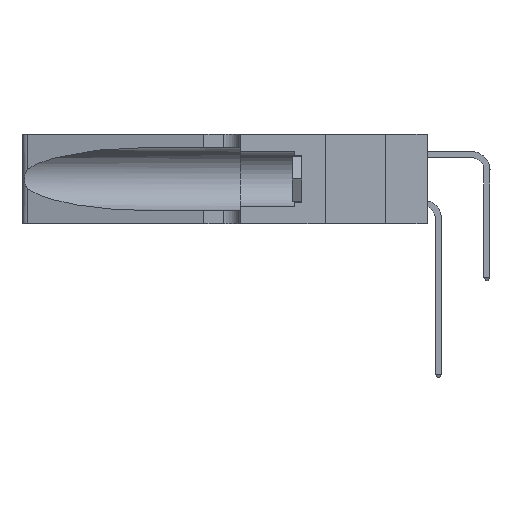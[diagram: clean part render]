
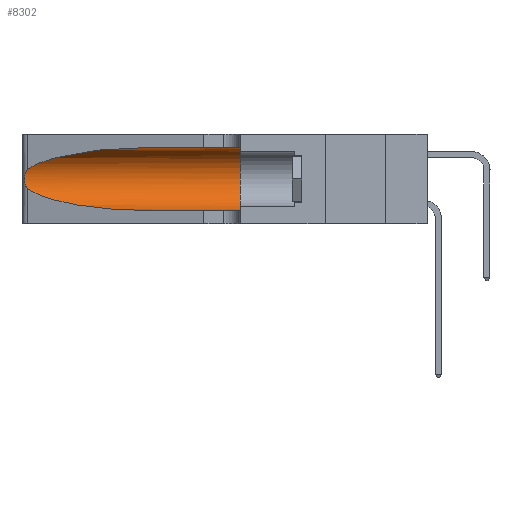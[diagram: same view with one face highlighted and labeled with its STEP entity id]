
A CAD part, left-side view. The second image highlights one B-rep face of the part: STEP entity #8302.
In plain terms, the highlighted cylindrical face has radius 3.308 mm (diameter 6.617 mm), a partial arc.
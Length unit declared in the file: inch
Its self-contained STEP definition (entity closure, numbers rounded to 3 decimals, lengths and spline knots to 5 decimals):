
#265 = EDGE_CURVE ( 'NONE', #23849, #14265, #804, .T. ) ;
#804 = B_SPLINE_CURVE_WITH_KNOTS ( 'NONE', 3,
 ( #3368, #3269, #7591, #3452, #15651, #3082, #5908, #24803, #11977, #8037, #22617, #1766, #9772, #3623 ),
 .UNSPECIFIED., .F., .F.,
 ( 4, 2, 2, 2, 2, 2, 4 ),
 ( 0., 0.00027, 0.00053, 0.00107, 0.0016, 0.00187, 0.00214 ),
 .UNSPECIFIED. ) ;
#1164 = CARTESIAN_POINT ( 'NONE',  ( 0.25487, 1.22718, 0.14631 ) ) ;
#1192 = DIRECTION ( 'NONE',  ( 0., -1., 0. ) ) ;
#1671 =( BOUNDED_CURVE ( )  B_SPLINE_CURVE ( 3, ( #26950, #3852, #14055, #14253 ),
 .UNSPECIFIED., .F., .T. ) 
 B_SPLINE_CURVE_WITH_KNOTS ( ( 4, 4 ),
 ( 1.5708, 2.84003 ),
 .UNSPECIFIED. ) 
 CURVE ( )  GEOMETRIC_REPRESENTATION_ITEM ( )  RATIONAL_B_SPLINE_CURVE ( ( 1., 0.87, 0.87, 1. ) ) 
 REPRESENTATION_ITEM ( '' )  );
#1766 = CARTESIAN_POINT ( 'NONE',  ( 0.25639, 1.23186, 0.15144 ) ) ;
#2797 = DIRECTION ( 'NONE',  ( 0., -1., 0. ) ) ;
#3082 = CARTESIAN_POINT ( 'NONE',  ( 0.26018, 1.23835, 0.19895 ) ) ;
#3269 = CARTESIAN_POINT ( 'NONE',  ( 0.25555, 1.22994, 0.2215 ) ) ;
#3368 = CARTESIAN_POINT ( 'NONE',  ( 0.25487, 1.22718, 0.22369 ) ) ;
#3452 = CARTESIAN_POINT ( 'NONE',  ( 0.25787, 1.23484, 0.2124 ) ) ;
#3623 = CARTESIAN_POINT ( 'NONE',  ( 0.25487, 1.22718, 0.14631 ) ) ;
#3852 = CARTESIAN_POINT ( 'NONE',  ( 0.18966, 0.96281, 0.31525 ) ) ;
#4766 = CARTESIAN_POINT ( 'NONE',  ( 0.1305, 0.72297, 0.31525 ) ) ;
#5136 = EDGE_CURVE ( 'NONE', #15925, #10423, #9144, .T. ) ;
#5548 = DIRECTION ( 'NONE',  ( 0., -1., 0. ) ) ;
#5908 = CARTESIAN_POINT ( 'NONE',  ( 0.26075, 1.23896, 0.19203 ) ) ;
#5994 = CYLINDRICAL_SURFACE ( 'NONE', #14311, 0.13025 ) ;
#6439 = CARTESIAN_POINT ( 'NONE',  ( 0.25487, 1.22718, 0.22369 ) ) ;
#6598 = EDGE_CURVE ( 'NONE', #14265, #10697, #26381, .T. ) ;
#7128 = CARTESIAN_POINT ( 'NONE',  ( 0.1305, 1.61858, 0.05475 ) ) ;
#7591 = CARTESIAN_POINT ( 'NONE',  ( 0.25639, 1.23184, 0.21858 ) ) ;
#8037 = CARTESIAN_POINT ( 'NONE',  ( 0.25856, 1.23593, 0.16098 ) ) ;
#8302 = ADVANCED_FACE ( 'NONE', ( #24354 ), #5994, .F. ) ;
#8969 = DIRECTION ( 'NONE',  ( 0., 1., 0. ) ) ;
#8988 = EDGE_CURVE ( 'NONE', #13413, #15925, #23983, .T. ) ;
#9144 = CIRCLE ( 'NONE', #11967, 0.13025 ) ;
#9772 = CARTESIAN_POINT ( 'NONE',  ( 0.25555, 1.22993, 0.14849 ) ) ;
#9868 = DIRECTION ( 'NONE',  ( 0., 0., -1. ) ) ;
#10423 = VERTEX_POINT ( 'NONE', #21136 ) ;
#10697 = VERTEX_POINT ( 'NONE', #17449 ) ;
#10906 = EDGE_CURVE ( 'NONE', #10697, #10423, #22584, .T. ) ;
#10915 = ORIENTED_EDGE ( 'NONE', *, *, #5136, .F. ) ;
#11065 = DIRECTION ( 'NONE',  ( 0., 0., 1. ) ) ;
#11659 = CARTESIAN_POINT ( 'NONE',  ( 0.18966, 0.96281, 0.05475 ) ) ;
#11967 = AXIS2_PLACEMENT_3D ( 'NONE', #23696, #8969, #11065 ) ;
#11977 = CARTESIAN_POINT ( 'NONE',  ( 0.26017, 1.23833, 0.17102 ) ) ;
#13413 = VERTEX_POINT ( 'NONE', #4766 ) ;
#13703 = EDGE_LOOP ( 'NONE', ( #15768, #22100, #19362, #14363, #10915, #14039 ) ) ;
#13873 = CARTESIAN_POINT ( 'NONE',  ( 0.1305, 1.61858, 0.31525 ) ) ;
#14039 = ORIENTED_EDGE ( 'NONE', *, *, #8988, .F. ) ;
#14055 = CARTESIAN_POINT ( 'NONE',  ( 0.2373, 1.15595, 0.28018 ) ) ;
#14253 = CARTESIAN_POINT ( 'NONE',  ( 0.25487, 1.22718, 0.22369 ) ) ;
#14265 = VERTEX_POINT ( 'NONE', #1164 ) ;
#14311 = AXIS2_PLACEMENT_3D ( 'NONE', #20161, #5548, #9868 ) ;
#14363 = ORIENTED_EDGE ( 'NONE', *, *, #10906, .T. ) ;
#15598 = CARTESIAN_POINT ( 'NONE',  ( 0.25487, 1.22718, 0.14631 ) ) ;
#15651 = CARTESIAN_POINT ( 'NONE',  ( 0.25854, 1.2359, 0.20912 ) ) ;
#15768 = ORIENTED_EDGE ( 'NONE', *, *, #23073, .T. ) ;
#15925 = VERTEX_POINT ( 'NONE', #24292 ) ;
#17449 = CARTESIAN_POINT ( 'NONE',  ( 0.1305, 0.72297, 0.05475 ) ) ;
#18067 = CARTESIAN_POINT ( 'NONE',  ( 0.1305, 0.72297, 0.05475 ) ) ;
#19362 = ORIENTED_EDGE ( 'NONE', *, *, #6598, .T. ) ;
#19957 = VECTOR ( 'NONE', #2797, 39.37008 ) ;
#20161 = CARTESIAN_POINT ( 'NONE',  ( 0.1305, 1.61858, 0.185 ) ) ;
#21136 = CARTESIAN_POINT ( 'NONE',  ( 0.1305, 0.35, 0.05475 ) ) ;
#21720 = VECTOR ( 'NONE', #1192, 39.37008 ) ;
#22100 = ORIENTED_EDGE ( 'NONE', *, *, #265, .T. ) ;
#22584 = LINE ( 'NONE', #7128, #19957 ) ;
#22617 = CARTESIAN_POINT ( 'NONE',  ( 0.25789, 1.23486, 0.15765 ) ) ;
#23073 = EDGE_CURVE ( 'NONE', #13413, #23849, #1671, .T. ) ;
#23696 = CARTESIAN_POINT ( 'NONE',  ( 0.1305, 0.35, 0.185 ) ) ;
#23849 = VERTEX_POINT ( 'NONE', #6439 ) ;
#23983 = LINE ( 'NONE', #13873, #21720 ) ;
#24292 = CARTESIAN_POINT ( 'NONE',  ( 0.1305, 0.35, 0.31525 ) ) ;
#24354 = FACE_OUTER_BOUND ( 'NONE', #13703, .T. ) ;
#24803 = CARTESIAN_POINT ( 'NONE',  ( 0.26075, 1.23896, 0.178 ) ) ;
#26201 = CARTESIAN_POINT ( 'NONE',  ( 0.2373, 1.15595, 0.08982 ) ) ;
#26381 =( BOUNDED_CURVE ( )  B_SPLINE_CURVE ( 3, ( #15598, #26201, #11659, #18067 ),
 .UNSPECIFIED., .F., .F. ) 
 B_SPLINE_CURVE_WITH_KNOTS ( ( 4, 4 ),
 ( 3.44316, 4.71239 ),
 .UNSPECIFIED. ) 
 CURVE ( )  GEOMETRIC_REPRESENTATION_ITEM ( )  RATIONAL_B_SPLINE_CURVE ( ( 1., 0.87, 0.87, 1. ) ) 
 REPRESENTATION_ITEM ( '' )  );
#26950 = CARTESIAN_POINT ( 'NONE',  ( 0.1305, 0.72297, 0.31525 ) ) ;
